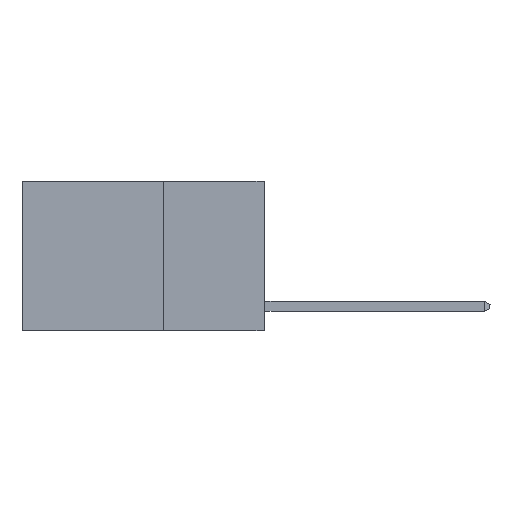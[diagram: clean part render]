
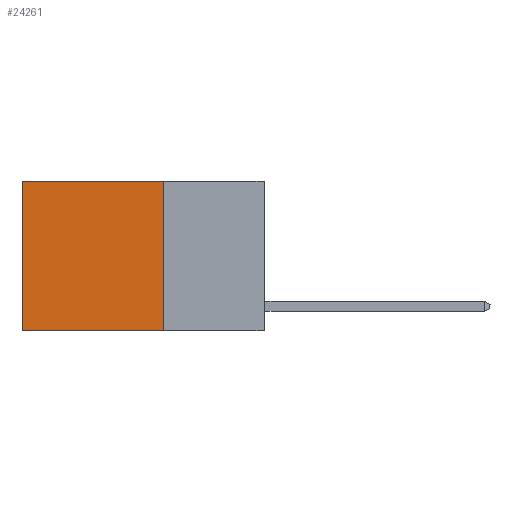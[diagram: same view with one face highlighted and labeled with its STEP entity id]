
A CAD part, left-side view. The second image highlights one B-rep face of the part: STEP entity #24261.
In plain terms, the highlighted planar face has unit normal (-1, 0, 0).
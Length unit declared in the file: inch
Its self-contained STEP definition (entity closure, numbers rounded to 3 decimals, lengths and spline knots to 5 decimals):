
#42 = EDGE_LOOP ( 'NONE', ( #23454, #23378, #19466, #20013 ) ) ;
#84 = VECTOR ( 'NONE', #5334, 39.37008 ) ;
#172 = DIRECTION ( 'NONE',  ( 0., 1., 0. ) ) ;
#198 = VECTOR ( 'NONE', #17780, 39.37008 ) ;
#857 = LINE ( 'NONE', #7928, #198 ) ;
#1219 = CARTESIAN_POINT ( 'NONE',  ( 0.2625, 0.25, 0. ) ) ;
#1675 = CARTESIAN_POINT ( 'NONE',  ( 0.2625, 0.6, -0.37 ) ) ;
#2161 = CARTESIAN_POINT ( 'NONE',  ( 0.2625, 0.25, -0.37 ) ) ;
#2667 = EDGE_CURVE ( 'NONE', #12227, #8180, #21576, .T. ) ;
#4801 = CARTESIAN_POINT ( 'NONE',  ( 0.2625, 0.25, -0.37 ) ) ;
#5334 = DIRECTION ( 'NONE',  ( 0., 0., -1. ) ) ;
#5530 = CARTESIAN_POINT ( 'NONE',  ( 0.2625, 0.25, 0. ) ) ;
#5615 = PLANE ( 'NONE',  #14166 ) ;
#7073 = EDGE_CURVE ( 'NONE', #11104, #9697, #857, .T. ) ;
#7585 = DIRECTION ( 'NONE',  ( 1., 0., 0. ) ) ;
#7928 = CARTESIAN_POINT ( 'NONE',  ( 0.2625, 0.25, 0. ) ) ;
#8180 = VERTEX_POINT ( 'NONE', #1675 ) ;
#9697 = VERTEX_POINT ( 'NONE', #4801 ) ;
#10193 = FACE_OUTER_BOUND ( 'NONE', #42, .T. ) ;
#10202 = DIRECTION ( 'NONE',  ( 0., 1., 0. ) ) ;
#10266 = CARTESIAN_POINT ( 'NONE',  ( 0.2625, 0.6, 0. ) ) ;
#11104 = VERTEX_POINT ( 'NONE', #1219 ) ;
#11127 = CARTESIAN_POINT ( 'NONE',  ( 0.2625, 0.6, 0. ) ) ;
#12122 = EDGE_CURVE ( 'NONE', #9697, #8180, #19515, .T. ) ;
#12227 = VERTEX_POINT ( 'NONE', #10266 ) ;
#14166 = AXIS2_PLACEMENT_3D ( 'NONE', #5530, #7585, #21219 ) ;
#17780 = DIRECTION ( 'NONE',  ( 0., 0., -1. ) ) ;
#18281 = VECTOR ( 'NONE', #172, 39.37008 ) ;
#19466 = ORIENTED_EDGE ( 'NONE', *, *, #7073, .F. ) ;
#19515 = LINE ( 'NONE', #2161, #18281 ) ;
#19973 = CARTESIAN_POINT ( 'NONE',  ( 0.2625, 0.25, 0. ) ) ;
#20013 = ORIENTED_EDGE ( 'NONE', *, *, #22700, .T. ) ;
#21219 = DIRECTION ( 'NONE',  ( 0., 0., -1. ) ) ;
#21566 = LINE ( 'NONE', #19973, #22164 ) ;
#21576 = LINE ( 'NONE', #11127, #84 ) ;
#22164 = VECTOR ( 'NONE', #10202, 39.37008 ) ;
#22700 = EDGE_CURVE ( 'NONE', #11104, #12227, #21566, .T. ) ;
#23378 = ORIENTED_EDGE ( 'NONE', *, *, #12122, .F. ) ;
#23454 = ORIENTED_EDGE ( 'NONE', *, *, #2667, .T. ) ;
#24261 = ADVANCED_FACE ( 'NONE', ( #10193 ), #5615, .F. ) ;
